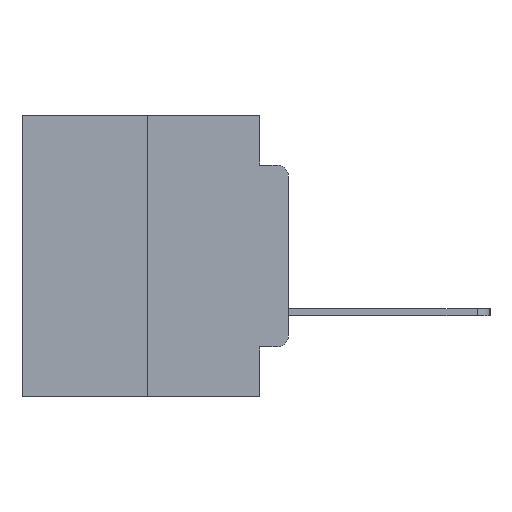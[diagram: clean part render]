
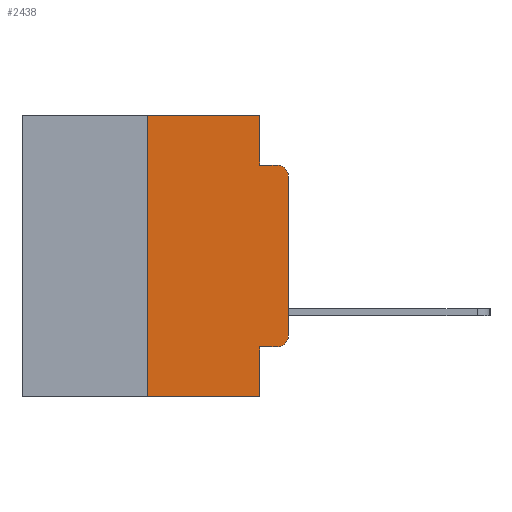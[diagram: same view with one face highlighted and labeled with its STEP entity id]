
A CAD part, left-side view. The second image highlights one B-rep face of the part: STEP entity #2438.
In plain terms, the highlighted planar face has unit normal (-1, 0, 0).
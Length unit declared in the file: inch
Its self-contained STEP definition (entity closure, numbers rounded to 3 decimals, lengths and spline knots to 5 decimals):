
#442 = CARTESIAN_POINT ( 'NONE',  ( 0., 0.051, -0.4115 ) ) ;
#594 = CARTESIAN_POINT ( 'NONE',  ( 0., 0.02, -0.0885 ) ) ;
#613 = VECTOR ( 'NONE', #1813, 39.37008 ) ;
#647 = CARTESIAN_POINT ( 'NONE',  ( 0., 0.02, -0.4115 ) ) ;
#709 = CIRCLE ( 'NONE', #20327, 0.02 ) ;
#865 = DIRECTION ( 'NONE',  ( 0., 0., 1. ) ) ;
#1813 = DIRECTION ( 'NONE',  ( 0., -1., 0. ) ) ;
#1907 = VERTEX_POINT ( 'NONE', #5387 ) ;
#2180 = AXIS2_PLACEMENT_3D ( 'NONE', #20343, #8816, #22237 ) ;
#2438 = ADVANCED_FACE ( 'NONE', ( #14387 ), #16371, .F. ) ;
#3004 = VECTOR ( 'NONE', #7164, 39.37008 ) ;
#3077 = LINE ( 'NONE', #442, #13242 ) ;
#3151 = VERTEX_POINT ( 'NONE', #15785 ) ;
#3262 = ORIENTED_EDGE ( 'NONE', *, *, #20402, .T. ) ;
#3938 = ORIENTED_EDGE ( 'NONE', *, *, #6875, .T. ) ;
#4294 = ORIENTED_EDGE ( 'NONE', *, *, #5166, .F. ) ;
#5086 = EDGE_CURVE ( 'NONE', #1907, #12222, #8288, .T. ) ;
#5089 = CARTESIAN_POINT ( 'NONE',  ( 0., 0., 0. ) ) ;
#5166 = EDGE_CURVE ( 'NONE', #21171, #12222, #20670, .T. ) ;
#5255 = VECTOR ( 'NONE', #865, 39.37008 ) ;
#5387 = CARTESIAN_POINT ( 'NONE',  ( 0., 0.25, -0.5 ) ) ;
#6133 = CARTESIAN_POINT ( 'NONE',  ( 0., 0.02, -0.3915 ) ) ;
#6187 = DIRECTION ( 'NONE',  ( 0., 0., -1. ) ) ;
#6547 = EDGE_CURVE ( 'NONE', #1907, #14570, #20870, .T. ) ;
#6819 = VECTOR ( 'NONE', #17521, 39.37008 ) ;
#6875 = EDGE_CURVE ( 'NONE', #3151, #7470, #7194, .T. ) ;
#7148 = CARTESIAN_POINT ( 'NONE',  ( 0., 0.473, 0. ) ) ;
#7164 = DIRECTION ( 'NONE',  ( 0., 0., 1. ) ) ;
#7194 = CIRCLE ( 'NONE', #2180, 0.02 ) ;
#7470 = VERTEX_POINT ( 'NONE', #594 ) ;
#8112 = CARTESIAN_POINT ( 'NONE',  ( 0., 0.051, -0.0885 ) ) ;
#8204 = DIRECTION ( 'NONE',  ( 0., 0., -1. ) ) ;
#8288 = LINE ( 'NONE', #21418, #17929 ) ;
#8526 = ORIENTED_EDGE ( 'NONE', *, *, #5086, .T. ) ;
#8816 = DIRECTION ( 'NONE',  ( -1., 0., 0. ) ) ;
#9063 = VECTOR ( 'NONE', #11399, 39.37008 ) ;
#10307 = CARTESIAN_POINT ( 'NONE',  ( 0., 0.051, 0. ) ) ;
#10717 = ORIENTED_EDGE ( 'NONE', *, *, #14230, .F. ) ;
#11399 = DIRECTION ( 'NONE',  ( 0., -1., 0. ) ) ;
#12222 = VERTEX_POINT ( 'NONE', #15575 ) ;
#12394 = VERTEX_POINT ( 'NONE', #19864 ) ;
#12416 = CARTESIAN_POINT ( 'NONE',  ( 0., 0.051, -0.0885 ) ) ;
#13242 = VECTOR ( 'NONE', #18412, 39.37008 ) ;
#13701 = EDGE_CURVE ( 'NONE', #12394, #13920, #18991, .T. ) ;
#13920 = VERTEX_POINT ( 'NONE', #12416 ) ;
#14230 = EDGE_CURVE ( 'NONE', #14570, #12394, #25412, .T. ) ;
#14357 = LINE ( 'NONE', #5089, #3004 ) ;
#14387 = FACE_OUTER_BOUND ( 'NONE', #16601, .T. ) ;
#14570 = VERTEX_POINT ( 'NONE', #16161 ) ;
#14658 = VERTEX_POINT ( 'NONE', #22193 ) ;
#14895 = ORIENTED_EDGE ( 'NONE', *, *, #21843, .T. ) ;
#15169 = ORIENTED_EDGE ( 'NONE', *, *, #13701, .F. ) ;
#15544 = VECTOR ( 'NONE', #6187, 39.37008 ) ;
#15575 = CARTESIAN_POINT ( 'NONE',  ( 0., 0.051, -0.5 ) ) ;
#15625 = CARTESIAN_POINT ( 'NONE',  ( 0., 0.051, 0. ) ) ;
#15785 = CARTESIAN_POINT ( 'NONE',  ( 0., 0., -0.1085 ) ) ;
#16161 = CARTESIAN_POINT ( 'NONE',  ( 0., 0.25, 0. ) ) ;
#16371 = PLANE ( 'NONE',  #21433 ) ;
#16526 = CARTESIAN_POINT ( 'NONE',  ( 0., 0.473, 0. ) ) ;
#16601 = EDGE_LOOP ( 'NONE', ( #3262, #3938, #24656, #15169, #10717, #16964, #8526, #4294, #14895, #23530 ) ) ;
#16774 = DIRECTION ( 'NONE',  ( 0., 0., -1. ) ) ;
#16899 = DIRECTION ( 'NONE',  ( 1., 0., 0. ) ) ;
#16935 = VERTEX_POINT ( 'NONE', #647 ) ;
#16964 = ORIENTED_EDGE ( 'NONE', *, *, #6547, .F. ) ;
#17521 = DIRECTION ( 'NONE',  ( 0., 0., -1. ) ) ;
#17926 = EDGE_CURVE ( 'NONE', #13920, #7470, #21135, .T. ) ;
#17929 = VECTOR ( 'NONE', #19508, 39.37008 ) ;
#18412 = DIRECTION ( 'NONE',  ( 0., -1., 0. ) ) ;
#18991 = LINE ( 'NONE', #15625, #6819 ) ;
#19508 = DIRECTION ( 'NONE',  ( 0., -1., 0. ) ) ;
#19795 = DIRECTION ( 'NONE',  ( -1., 0., 0. ) ) ;
#19864 = CARTESIAN_POINT ( 'NONE',  ( 0., 0.051, 0. ) ) ;
#20327 = AXIS2_PLACEMENT_3D ( 'NONE', #6133, #19795, #8204 ) ;
#20343 = CARTESIAN_POINT ( 'NONE',  ( 0., 0.02, -0.1085 ) ) ;
#20402 = EDGE_CURVE ( 'NONE', #14658, #3151, #14357, .T. ) ;
#20670 = LINE ( 'NONE', #10307, #15544 ) ;
#20795 = CARTESIAN_POINT ( 'NONE',  ( 0., 0.051, -0.4115 ) ) ;
#20870 = LINE ( 'NONE', #24445, #5255 ) ;
#21135 = LINE ( 'NONE', #8112, #613 ) ;
#21171 = VERTEX_POINT ( 'NONE', #20795 ) ;
#21418 = CARTESIAN_POINT ( 'NONE',  ( 0., 0.473, -0.5 ) ) ;
#21433 = AXIS2_PLACEMENT_3D ( 'NONE', #16526, #16899, #16774 ) ;
#21843 = EDGE_CURVE ( 'NONE', #21171, #16935, #3077, .T. ) ;
#22193 = CARTESIAN_POINT ( 'NONE',  ( 0., 0., -0.3915 ) ) ;
#22237 = DIRECTION ( 'NONE',  ( 0., 0., -1. ) ) ;
#23092 = EDGE_CURVE ( 'NONE', #16935, #14658, #709, .T. ) ;
#23530 = ORIENTED_EDGE ( 'NONE', *, *, #23092, .T. ) ;
#24445 = CARTESIAN_POINT ( 'NONE',  ( 0., 0.25, 0. ) ) ;
#24656 = ORIENTED_EDGE ( 'NONE', *, *, #17926, .F. ) ;
#25412 = LINE ( 'NONE', #7148, #9063 ) ;
